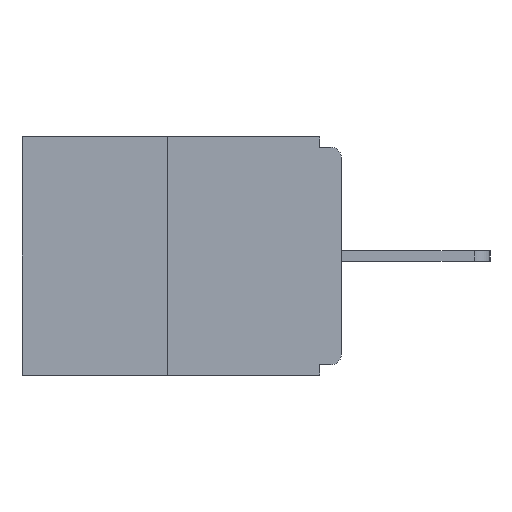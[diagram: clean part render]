
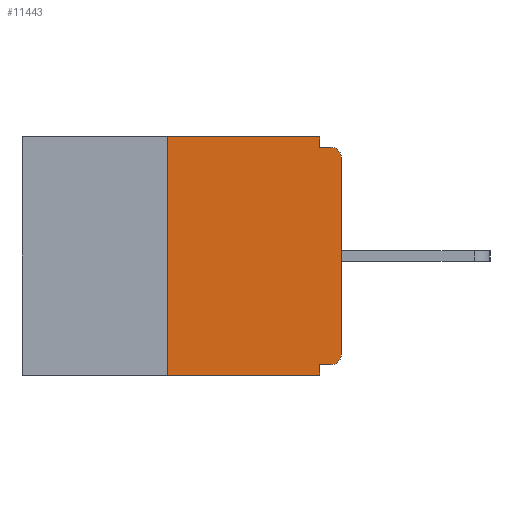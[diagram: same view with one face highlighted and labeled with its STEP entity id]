
A CAD part, left-side view. The second image highlights one B-rep face of the part: STEP entity #11443.
In plain terms, the highlighted planar face has unit normal (-1, 0, 0).
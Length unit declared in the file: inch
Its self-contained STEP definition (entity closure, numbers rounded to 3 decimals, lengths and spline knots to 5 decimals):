
#81 = ORIENTED_EDGE ( 'NONE', *, *, #15331, .F. ) ;
#532 = LINE ( 'NONE', #16147, #12717 ) ;
#778 = DIRECTION ( 'NONE',  ( 0., 1., 0. ) ) ;
#827 = CARTESIAN_POINT ( 'NONE',  ( 0., 0.25, 0. ) ) ;
#1223 = CARTESIAN_POINT ( 'NONE',  ( 0., 0., -0.03 ) ) ;
#1725 = CARTESIAN_POINT ( 'NONE',  ( 0., 0., -0.015 ) ) ;
#1757 = CARTESIAN_POINT ( 'NONE',  ( 0., 0.015, -0.313 ) ) ;
#1839 = CARTESIAN_POINT ( 'NONE',  ( 0., 0.46, 0. ) ) ;
#2408 = DIRECTION ( 'NONE',  ( -1., 0., 0. ) ) ;
#2440 = VERTEX_POINT ( 'NONE', #11379 ) ;
#2996 = VECTOR ( 'NONE', #778, 39.37008 ) ;
#3151 = EDGE_LOOP ( 'NONE', ( #7310, #7632, #9640, #81, #10533, #8246, #6476, #15702, #21508, #11879 ) ) ;
#3197 = DIRECTION ( 'NONE',  ( 0., -1., 0. ) ) ;
#3341 = DIRECTION ( 'NONE',  ( 1., 0., 0. ) ) ;
#3415 = AXIS2_PLACEMENT_3D ( 'NONE', #1757, #18870, #5489 ) ;
#3502 = EDGE_CURVE ( 'NONE', #20178, #2440, #9801, .T. ) ;
#3721 = FACE_OUTER_BOUND ( 'NONE', #3151, .T. ) ;
#3739 = VERTEX_POINT ( 'NONE', #1223 ) ;
#4239 = EDGE_CURVE ( 'NONE', #21152, #7080, #18559, .T. ) ;
#4976 = EDGE_CURVE ( 'NONE', #3739, #10159, #20780, .T. ) ;
#5251 = LINE ( 'NONE', #10892, #7189 ) ;
#5489 = DIRECTION ( 'NONE',  ( 0., 0., -1. ) ) ;
#6304 = VECTOR ( 'NONE', #17942, 39.37008 ) ;
#6476 = ORIENTED_EDGE ( 'NONE', *, *, #21964, .T. ) ;
#7013 = CARTESIAN_POINT ( 'NONE',  ( 0., 0.25, 0. ) ) ;
#7080 = VERTEX_POINT ( 'NONE', #24665 ) ;
#7189 = VECTOR ( 'NONE', #14764, 39.37008 ) ;
#7310 = ORIENTED_EDGE ( 'NONE', *, *, #10056, .F. ) ;
#7437 = CARTESIAN_POINT ( 'NONE',  ( 0., 0.46, -0.343 ) ) ;
#7632 = ORIENTED_EDGE ( 'NONE', *, *, #19761, .F. ) ;
#7721 = VERTEX_POINT ( 'NONE', #7013 ) ;
#8246 = ORIENTED_EDGE ( 'NONE', *, *, #3502, .T. ) ;
#8293 = CARTESIAN_POINT ( 'NONE',  ( 0., 0.015, -0.328 ) ) ;
#8313 = CARTESIAN_POINT ( 'NONE',  ( 0., 0.015, -0.015 ) ) ;
#8842 = CARTESIAN_POINT ( 'NONE',  ( 0., 0.46, 0. ) ) ;
#8885 = EDGE_CURVE ( 'NONE', #20178, #21556, #23872, .T. ) ;
#9219 = CARTESIAN_POINT ( 'NONE',  ( 0., 0.031, 0. ) ) ;
#9584 = LINE ( 'NONE', #1839, #16560 ) ;
#9640 = ORIENTED_EDGE ( 'NONE', *, *, #4239, .T. ) ;
#9801 = CIRCLE ( 'NONE', #3415, 0.015 ) ;
#10056 = EDGE_CURVE ( 'NONE', #7721, #11424, #9584, .T. ) ;
#10159 = VERTEX_POINT ( 'NONE', #8313 ) ;
#10338 = VECTOR ( 'NONE', #3197, 39.37008 ) ;
#10396 = AXIS2_PLACEMENT_3D ( 'NONE', #23745, #2408, #23494 ) ;
#10533 = ORIENTED_EDGE ( 'NONE', *, *, #8885, .F. ) ;
#10892 = CARTESIAN_POINT ( 'NONE',  ( 0., 0.031, -0.343 ) ) ;
#10975 = LINE ( 'NONE', #1725, #21119 ) ;
#11094 = PLANE ( 'NONE',  #13604 ) ;
#11379 = CARTESIAN_POINT ( 'NONE',  ( 0., 0., -0.313 ) ) ;
#11424 = VERTEX_POINT ( 'NONE', #9219 ) ;
#11443 = ADVANCED_FACE ( 'NONE', ( #3721 ), #11094, .F. ) ;
#11771 = VERTEX_POINT ( 'NONE', #23550 ) ;
#11879 = ORIENTED_EDGE ( 'NONE', *, *, #17713, .F. ) ;
#12717 = VECTOR ( 'NONE', #19642, 39.37008 ) ;
#13604 = AXIS2_PLACEMENT_3D ( 'NONE', #8842, #3341, #16596 ) ;
#13809 = DIRECTION ( 'NONE',  ( 0., 0., -1. ) ) ;
#14059 = CARTESIAN_POINT ( 'NONE',  ( 0., 0.031, 0. ) ) ;
#14764 = DIRECTION ( 'NONE',  ( 0., 0., -1. ) ) ;
#15331 = EDGE_CURVE ( 'NONE', #21556, #7080, #5251, .T. ) ;
#15702 = ORIENTED_EDGE ( 'NONE', *, *, #4976, .T. ) ;
#16147 = CARTESIAN_POINT ( 'NONE',  ( 0., 0., 0. ) ) ;
#16272 = CARTESIAN_POINT ( 'NONE',  ( 0., 0., -0.328 ) ) ;
#16560 = VECTOR ( 'NONE', #24557, 39.37008 ) ;
#16596 = DIRECTION ( 'NONE',  ( 0., 0., -1. ) ) ;
#17713 = EDGE_CURVE ( 'NONE', #11424, #11771, #17805, .T. ) ;
#17805 = LINE ( 'NONE', #14059, #18737 ) ;
#17942 = DIRECTION ( 'NONE',  ( 0., 0., 1. ) ) ;
#18559 = LINE ( 'NONE', #7437, #10338 ) ;
#18583 = DIRECTION ( 'NONE',  ( 0., -1., 0. ) ) ;
#18737 = VECTOR ( 'NONE', #13809, 39.37008 ) ;
#18870 = DIRECTION ( 'NONE',  ( -1., 0., 0. ) ) ;
#19642 = DIRECTION ( 'NONE',  ( 0., 0., 1. ) ) ;
#19761 = EDGE_CURVE ( 'NONE', #21152, #7721, #23916, .T. ) ;
#20178 = VERTEX_POINT ( 'NONE', #8293 ) ;
#20780 = CIRCLE ( 'NONE', #10396, 0.015 ) ;
#21119 = VECTOR ( 'NONE', #18583, 39.37008 ) ;
#21152 = VERTEX_POINT ( 'NONE', #21363 ) ;
#21222 = CARTESIAN_POINT ( 'NONE',  ( 0., 0.031, -0.328 ) ) ;
#21363 = CARTESIAN_POINT ( 'NONE',  ( 0., 0.25, -0.343 ) ) ;
#21508 = ORIENTED_EDGE ( 'NONE', *, *, #22355, .F. ) ;
#21556 = VERTEX_POINT ( 'NONE', #21222 ) ;
#21964 = EDGE_CURVE ( 'NONE', #2440, #3739, #532, .T. ) ;
#22355 = EDGE_CURVE ( 'NONE', #11771, #10159, #10975, .T. ) ;
#23494 = DIRECTION ( 'NONE',  ( 0., 0., -1. ) ) ;
#23550 = CARTESIAN_POINT ( 'NONE',  ( 0., 0.031, -0.015 ) ) ;
#23745 = CARTESIAN_POINT ( 'NONE',  ( 0., 0.015, -0.03 ) ) ;
#23872 = LINE ( 'NONE', #16272, #2996 ) ;
#23916 = LINE ( 'NONE', #827, #6304 ) ;
#24557 = DIRECTION ( 'NONE',  ( 0., -1., 0. ) ) ;
#24665 = CARTESIAN_POINT ( 'NONE',  ( 0., 0.031, -0.343 ) ) ;
